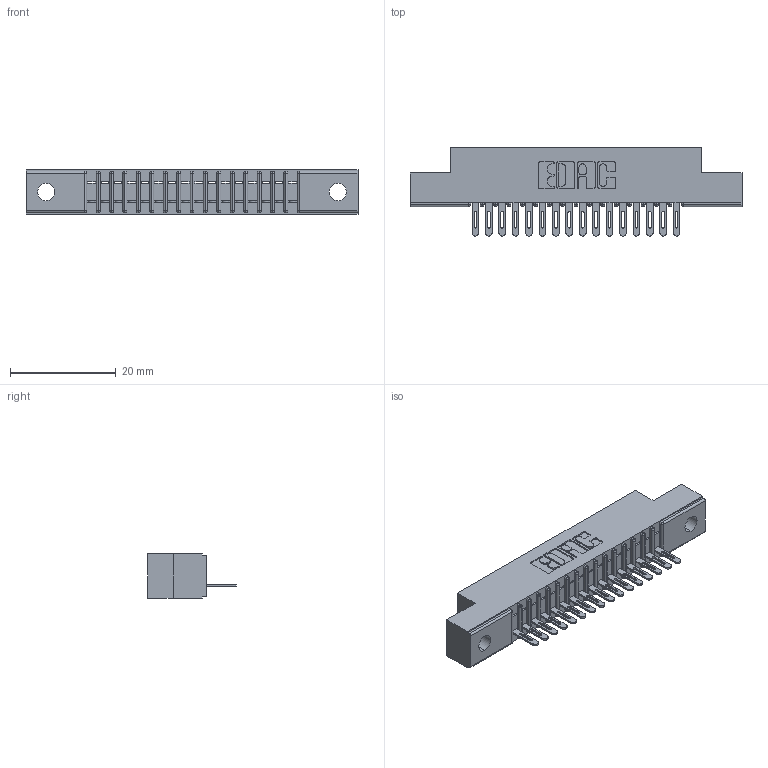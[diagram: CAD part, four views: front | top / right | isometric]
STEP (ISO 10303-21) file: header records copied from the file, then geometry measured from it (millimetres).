
FILE_DESCRIPTION (( 'STEP AP203' ), '1' );
FILE_NAME ('341-016-500-102.STEP', '2018-08-06T15:31:19', ( '' ), ( '' ), 'SwSTEP 2.0', 'SolidWorks 2016', '' );
FILE_SCHEMA (( 'CONFIG_CONTROL_DESIGN' ));
Length unit declared in the file: inch
Products named in the file (3): 341-016-500-102; 341 Part_.128 (3.25) Dia Mounting Holes; 341-292-001_341-292-100
Assembly tree (17 placements, depth 2):
  341-016-500-102
    341 Part_.128 (3.25) Dia Mounting Holes
    341-292-001_341-292-100  x16
Bounding box: 62.87 x 16.69 x 8.38 mm (x, y, z)
Volume: 3461.4 mm3; surface area: 5966.9 mm2
Topology: 17 solids, 17 shells, 1428 faces, 4108 edges, 2638 vertices
Faces by surface type: plane 852, cylinder 512, sphere 34, torus 30
Entity records: 22325 total; most frequent: CARTESIAN_POINT 3780, ORIENTED_EDGE 3768, DIRECTION 3674, EDGE_CURVE 1884, LINE 1490, VECTOR 1490, VERTEX_POINT 1198, AXIS2_PLACEMENT_3D 1092
